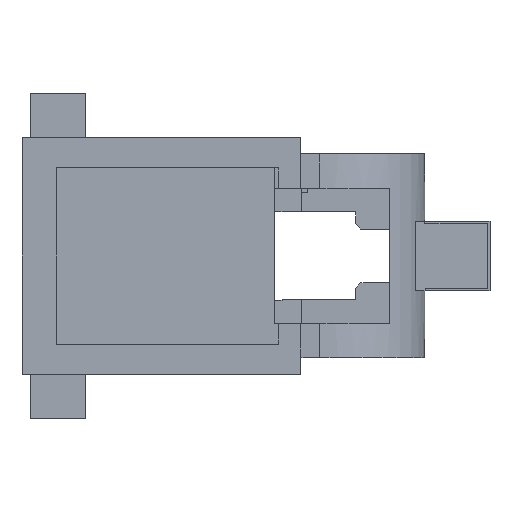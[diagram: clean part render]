
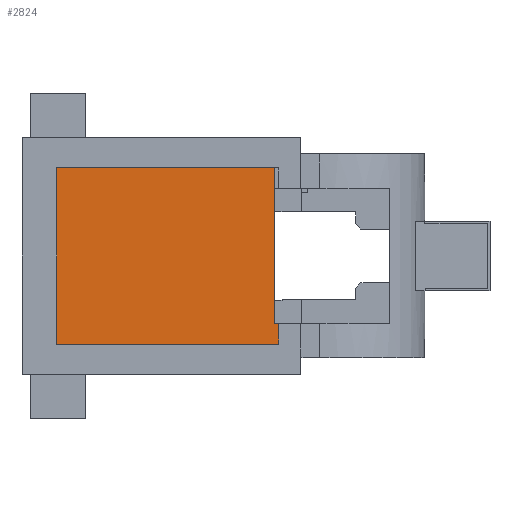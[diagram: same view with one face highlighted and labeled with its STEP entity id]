
A CAD part, left-side view. The second image highlights one B-rep face of the part: STEP entity #2824.
In plain terms, the highlighted planar face has unit normal (-1, 0, 0).
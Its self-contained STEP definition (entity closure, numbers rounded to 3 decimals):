
#642 = PLANE('',#643);
#643 = AXIS2_PLACEMENT_3D('',#644,#645,#646);
#644 = CARTESIAN_POINT('',(-69.606,33.68,21.5));
#645 = DIRECTION('',(0.,-1.,0.));
#646 = DIRECTION('',(1.,0.,0.));
#782 = PLANE('',#783);
#783 = AXIS2_PLACEMENT_3D('',#784,#785,#786);
#784 = CARTESIAN_POINT('',(-177.8,73.213,16.));
#785 = DIRECTION('',(0.,0.,-1.));
#786 = DIRECTION('',(0.,-1.,0.));
#1226 = VERTEX_POINT('',#1227);
#1227 = CARTESIAN_POINT('',(-25.8,33.68,12.218));
#1240 = PLANE('',#1241);
#1241 = AXIS2_PLACEMENT_3D('',#1242,#1243,#1244);
#1242 = CARTESIAN_POINT('',(-177.8,33.7,12.218));
#1243 = DIRECTION('',(0.,0.,-1.));
#1244 = DIRECTION('',(0.,-1.,0.));
#1303 = VERTEX_POINT('',#1304);
#1304 = CARTESIAN_POINT('',(-25.8,33.68,16.));
#1323 = EDGE_CURVE('',#1226,#1303,#1324,.T.);
#1324 = SURFACE_CURVE('',#1325,(#1329,#1335),.PCURVE_S1.);
#1325 = LINE('',#1326,#1327);
#1326 = CARTESIAN_POINT('',(-25.8,33.68,18.75));
#1327 = VECTOR('',#1328,1.);
#1328 = DIRECTION('',(0.,0.,1.));
#1329 = PCURVE('',#642,#1330);
#1330 = DEFINITIONAL_REPRESENTATION('',(#1331),#1334);
#1331 = B_SPLINE_CURVE_WITH_KNOTS('',1,(#1332,#1333),.UNSPECIFIED.,.F.,
  .F.,(2,2),(-7.25,-2.75),.PIECEWISE_BEZIER_KNOTS.);
#1332 = CARTESIAN_POINT('',(43.806,-10.));
#1333 = CARTESIAN_POINT('',(43.806,-5.5));
#1334 = ( GEOMETRIC_REPRESENTATION_CONTEXT(2) 
PARAMETRIC_REPRESENTATION_CONTEXT() REPRESENTATION_CONTEXT('2D SPACE',''
  ) );
#1335 = PCURVE('',#1336,#1341);
#1336 = PLANE('',#1337);
#1337 = AXIS2_PLACEMENT_3D('',#1338,#1339,#1340);
#1338 = CARTESIAN_POINT('',(-25.8,73.213,16.));
#1339 = DIRECTION('',(-1.,0.,0.));
#1340 = DIRECTION('',(0.,0.,-1.));
#1341 = DEFINITIONAL_REPRESENTATION('',(#1342),#1345);
#1342 = B_SPLINE_CURVE_WITH_KNOTS('',1,(#1343,#1344),.UNSPECIFIED.,.F.,
  .F.,(2,2),(-7.25,-2.75),.PIECEWISE_BEZIER_KNOTS.);
#1343 = CARTESIAN_POINT('',(4.5,39.533));
#1344 = CARTESIAN_POINT('',(0.,39.533));
#1345 = ( GEOMETRIC_REPRESENTATION_CONTEXT(2) 
PARAMETRIC_REPRESENTATION_CONTEXT() REPRESENTATION_CONTEXT('2D SPACE',''
  ) );
#1391 = PLANE('',#1392);
#1392 = AXIS2_PLACEMENT_3D('',#1393,#1394,#1395);
#1393 = CARTESIAN_POINT('',(-177.8,73.213,-16.));
#1394 = DIRECTION('',(0.,-1.,0.));
#1395 = DIRECTION('',(0.,0.,1.));
#1419 = PLANE('',#1420);
#1420 = AXIS2_PLACEMENT_3D('',#1421,#1422,#1423);
#1421 = CARTESIAN_POINT('',(-177.8,32.852,-16.));
#1422 = DIRECTION('',(0.,0.,1.));
#1423 = DIRECTION('',(0.,1.,0.));
#1447 = PLANE('',#1448);
#1448 = AXIS2_PLACEMENT_3D('',#1449,#1450,#1451);
#1449 = CARTESIAN_POINT('',(-177.8,32.852,16.));
#1450 = DIRECTION('',(0.,1.,0.));
#1451 = DIRECTION('',(0.,0.,-1.));
#1475 = PLANE('',#1476);
#1476 = AXIS2_PLACEMENT_3D('',#1477,#1478,#1479);
#1477 = CARTESIAN_POINT('',(-177.8,28.825,-12.276));
#1478 = DIRECTION('',(0.,0.,1.));
#1479 = DIRECTION('',(0.,1.,0.));
#1936 = EDGE_CURVE('',#1937,#1303,#1939,.T.);
#1937 = VERTEX_POINT('',#1938);
#1938 = CARTESIAN_POINT('',(-25.8,73.213,16.));
#1939 = SURFACE_CURVE('',#1940,(#1944,#1951),.PCURVE_S1.);
#1940 = LINE('',#1941,#1942);
#1941 = CARTESIAN_POINT('',(-25.8,73.213,16.));
#1942 = VECTOR('',#1943,1.);
#1943 = DIRECTION('',(0.,-1.,0.));
#1944 = PCURVE('',#782,#1945);
#1945 = DEFINITIONAL_REPRESENTATION('',(#1946),#1950);
#1946 = LINE('',#1947,#1948);
#1947 = CARTESIAN_POINT('',(0.,-152.));
#1948 = VECTOR('',#1949,1.);
#1949 = DIRECTION('',(1.,0.));
#1950 = ( GEOMETRIC_REPRESENTATION_CONTEXT(2) 
PARAMETRIC_REPRESENTATION_CONTEXT() REPRESENTATION_CONTEXT('2D SPACE',''
  ) );
#1951 = PCURVE('',#1336,#1952);
#1952 = DEFINITIONAL_REPRESENTATION('',(#1953),#1957);
#1953 = LINE('',#1954,#1955);
#1954 = CARTESIAN_POINT('',(0.,0.));
#1955 = VECTOR('',#1956,1.);
#1956 = DIRECTION('',(0.,1.));
#1957 = ( GEOMETRIC_REPRESENTATION_CONTEXT(2) 
PARAMETRIC_REPRESENTATION_CONTEXT() REPRESENTATION_CONTEXT('2D SPACE',''
  ) );
#2701 = EDGE_CURVE('',#2702,#1226,#2704,.T.);
#2702 = VERTEX_POINT('',#2703);
#2703 = CARTESIAN_POINT('',(-25.8,33.7,12.218));
#2704 = SURFACE_CURVE('',#2705,(#2709,#2715),.PCURVE_S1.);
#2705 = LINE('',#2706,#2707);
#2706 = CARTESIAN_POINT('',(-25.8,53.456,12.218));
#2707 = VECTOR('',#2708,1.);
#2708 = DIRECTION('',(0.,-1.,0.));
#2709 = PCURVE('',#1240,#2710);
#2710 = DEFINITIONAL_REPRESENTATION('',(#2711),#2714);
#2711 = B_SPLINE_CURVE_WITH_KNOTS('',1,(#2712,#2713),.UNSPECIFIED.,.F.,
  .F.,(2,2),(19.756,20.604),.PIECEWISE_BEZIER_KNOTS.);
#2712 = CARTESIAN_POINT('',(0.,-152.));
#2713 = CARTESIAN_POINT('',(0.848,-152.));
#2714 = ( GEOMETRIC_REPRESENTATION_CONTEXT(2) 
PARAMETRIC_REPRESENTATION_CONTEXT() REPRESENTATION_CONTEXT('2D SPACE',''
  ) );
#2715 = PCURVE('',#1336,#2716);
#2716 = DEFINITIONAL_REPRESENTATION('',(#2717),#2720);
#2717 = B_SPLINE_CURVE_WITH_KNOTS('',1,(#2718,#2719),.UNSPECIFIED.,.F.,
  .F.,(2,2),(19.756,20.604),.PIECEWISE_BEZIER_KNOTS.);
#2718 = CARTESIAN_POINT('',(3.782,39.513));
#2719 = CARTESIAN_POINT('',(3.782,40.361));
#2720 = ( GEOMETRIC_REPRESENTATION_CONTEXT(2) 
PARAMETRIC_REPRESENTATION_CONTEXT() REPRESENTATION_CONTEXT('2D SPACE',''
  ) );
#2738 = PLANE('',#2739);
#2739 = AXIS2_PLACEMENT_3D('',#2740,#2741,#2742);
#2740 = CARTESIAN_POINT('',(-177.8,33.7,-12.276));
#2741 = DIRECTION('',(0.,-1.,0.));
#2742 = DIRECTION('',(0.,0.,1.));
#2824 = ADVANCED_FACE('',(#2825),#1336,.T.);
#2825 = FACE_BOUND('',#2826,.T.);
#2826 = EDGE_LOOP('',(#2827,#2828,#2829,#2830,#2853,#2876,#2899,#2920));
#2827 = ORIENTED_EDGE('',*,*,#2701,.T.);
#2828 = ORIENTED_EDGE('',*,*,#1323,.T.);
#2829 = ORIENTED_EDGE('',*,*,#1936,.F.);
#2830 = ORIENTED_EDGE('',*,*,#2831,.F.);
#2831 = EDGE_CURVE('',#2832,#1937,#2834,.T.);
#2832 = VERTEX_POINT('',#2833);
#2833 = CARTESIAN_POINT('',(-25.8,73.213,-16.));
#2834 = SURFACE_CURVE('',#2835,(#2839,#2846),.PCURVE_S1.);
#2835 = LINE('',#2836,#2837);
#2836 = CARTESIAN_POINT('',(-25.8,73.213,-16.));
#2837 = VECTOR('',#2838,1.);
#2838 = DIRECTION('',(0.,0.,1.));
#2839 = PCURVE('',#1336,#2840);
#2840 = DEFINITIONAL_REPRESENTATION('',(#2841),#2845);
#2841 = LINE('',#2842,#2843);
#2842 = CARTESIAN_POINT('',(32.,0.));
#2843 = VECTOR('',#2844,1.);
#2844 = DIRECTION('',(-1.,0.));
#2845 = ( GEOMETRIC_REPRESENTATION_CONTEXT(2) 
PARAMETRIC_REPRESENTATION_CONTEXT() REPRESENTATION_CONTEXT('2D SPACE',''
  ) );
#2846 = PCURVE('',#1391,#2847);
#2847 = DEFINITIONAL_REPRESENTATION('',(#2848),#2852);
#2848 = LINE('',#2849,#2850);
#2849 = CARTESIAN_POINT('',(0.,-152.));
#2850 = VECTOR('',#2851,1.);
#2851 = DIRECTION('',(1.,0.));
#2852 = ( GEOMETRIC_REPRESENTATION_CONTEXT(2) 
PARAMETRIC_REPRESENTATION_CONTEXT() REPRESENTATION_CONTEXT('2D SPACE',''
  ) );
#2853 = ORIENTED_EDGE('',*,*,#2854,.F.);
#2854 = EDGE_CURVE('',#2855,#2832,#2857,.T.);
#2855 = VERTEX_POINT('',#2856);
#2856 = CARTESIAN_POINT('',(-25.8,32.852,-16.));
#2857 = SURFACE_CURVE('',#2858,(#2862,#2869),.PCURVE_S1.);
#2858 = LINE('',#2859,#2860);
#2859 = CARTESIAN_POINT('',(-25.8,32.852,-16.));
#2860 = VECTOR('',#2861,1.);
#2861 = DIRECTION('',(0.,1.,0.));
#2862 = PCURVE('',#1336,#2863);
#2863 = DEFINITIONAL_REPRESENTATION('',(#2864),#2868);
#2864 = LINE('',#2865,#2866);
#2865 = CARTESIAN_POINT('',(32.,40.361));
#2866 = VECTOR('',#2867,1.);
#2867 = DIRECTION('',(0.,-1.));
#2868 = ( GEOMETRIC_REPRESENTATION_CONTEXT(2) 
PARAMETRIC_REPRESENTATION_CONTEXT() REPRESENTATION_CONTEXT('2D SPACE',''
  ) );
#2869 = PCURVE('',#1419,#2870);
#2870 = DEFINITIONAL_REPRESENTATION('',(#2871),#2875);
#2871 = LINE('',#2872,#2873);
#2872 = CARTESIAN_POINT('',(0.,-152.));
#2873 = VECTOR('',#2874,1.);
#2874 = DIRECTION('',(1.,0.));
#2875 = ( GEOMETRIC_REPRESENTATION_CONTEXT(2) 
PARAMETRIC_REPRESENTATION_CONTEXT() REPRESENTATION_CONTEXT('2D SPACE',''
  ) );
#2876 = ORIENTED_EDGE('',*,*,#2877,.F.);
#2877 = EDGE_CURVE('',#2878,#2855,#2880,.T.);
#2878 = VERTEX_POINT('',#2879);
#2879 = CARTESIAN_POINT('',(-25.8,32.852,-12.276));
#2880 = SURFACE_CURVE('',#2881,(#2885,#2892),.PCURVE_S1.);
#2881 = LINE('',#2882,#2883);
#2882 = CARTESIAN_POINT('',(-25.8,32.852,16.));
#2883 = VECTOR('',#2884,1.);
#2884 = DIRECTION('',(0.,0.,-1.));
#2885 = PCURVE('',#1336,#2886);
#2886 = DEFINITIONAL_REPRESENTATION('',(#2887),#2891);
#2887 = LINE('',#2888,#2889);
#2888 = CARTESIAN_POINT('',(0.,40.361));
#2889 = VECTOR('',#2890,1.);
#2890 = DIRECTION('',(1.,0.));
#2891 = ( GEOMETRIC_REPRESENTATION_CONTEXT(2) 
PARAMETRIC_REPRESENTATION_CONTEXT() REPRESENTATION_CONTEXT('2D SPACE',''
  ) );
#2892 = PCURVE('',#1447,#2893);
#2893 = DEFINITIONAL_REPRESENTATION('',(#2894),#2898);
#2894 = LINE('',#2895,#2896);
#2895 = CARTESIAN_POINT('',(0.,-152.));
#2896 = VECTOR('',#2897,1.);
#2897 = DIRECTION('',(1.,0.));
#2898 = ( GEOMETRIC_REPRESENTATION_CONTEXT(2) 
PARAMETRIC_REPRESENTATION_CONTEXT() REPRESENTATION_CONTEXT('2D SPACE',''
  ) );
#2899 = ORIENTED_EDGE('',*,*,#2900,.T.);
#2900 = EDGE_CURVE('',#2878,#2901,#2903,.T.);
#2901 = VERTEX_POINT('',#2902);
#2902 = CARTESIAN_POINT('',(-25.8,33.7,-12.276));
#2903 = SURFACE_CURVE('',#2904,(#2908,#2914),.PCURVE_S1.);
#2904 = LINE('',#2905,#2906);
#2905 = CARTESIAN_POINT('',(-25.8,51.019,-12.276));
#2906 = VECTOR('',#2907,1.);
#2907 = DIRECTION('',(0.,1.,0.));
#2908 = PCURVE('',#1336,#2909);
#2909 = DEFINITIONAL_REPRESENTATION('',(#2910),#2913);
#2910 = B_SPLINE_CURVE_WITH_KNOTS('',1,(#2911,#2912),.UNSPECIFIED.,.F.,
  .F.,(2,2),(-18.167,-17.319),.PIECEWISE_BEZIER_KNOTS.);
#2911 = CARTESIAN_POINT('',(28.276,40.361));
#2912 = CARTESIAN_POINT('',(28.276,39.513));
#2913 = ( GEOMETRIC_REPRESENTATION_CONTEXT(2) 
PARAMETRIC_REPRESENTATION_CONTEXT() REPRESENTATION_CONTEXT('2D SPACE',''
  ) );
#2914 = PCURVE('',#1475,#2915);
#2915 = DEFINITIONAL_REPRESENTATION('',(#2916),#2919);
#2916 = B_SPLINE_CURVE_WITH_KNOTS('',1,(#2917,#2918),.UNSPECIFIED.,.F.,
  .F.,(2,2),(-18.167,-17.319),.PIECEWISE_BEZIER_KNOTS.);
#2917 = CARTESIAN_POINT('',(4.027,-152.));
#2918 = CARTESIAN_POINT('',(4.875,-152.));
#2919 = ( GEOMETRIC_REPRESENTATION_CONTEXT(2) 
PARAMETRIC_REPRESENTATION_CONTEXT() REPRESENTATION_CONTEXT('2D SPACE',''
  ) );
#2920 = ORIENTED_EDGE('',*,*,#2921,.T.);
#2921 = EDGE_CURVE('',#2901,#2702,#2922,.T.);
#2922 = SURFACE_CURVE('',#2923,(#2927,#2933),.PCURVE_S1.);
#2923 = LINE('',#2924,#2925);
#2924 = CARTESIAN_POINT('',(-25.8,33.7,1.862));
#2925 = VECTOR('',#2926,1.);
#2926 = DIRECTION('',(0.,0.,1.));
#2927 = PCURVE('',#1336,#2928);
#2928 = DEFINITIONAL_REPRESENTATION('',(#2929),#2932);
#2929 = B_SPLINE_CURVE_WITH_KNOTS('',1,(#2930,#2931),.UNSPECIFIED.,.F.,
  .F.,(2,2),(-14.138,10.356),.PIECEWISE_BEZIER_KNOTS.);
#2930 = CARTESIAN_POINT('',(28.276,39.513));
#2931 = CARTESIAN_POINT('',(3.782,39.513));
#2932 = ( GEOMETRIC_REPRESENTATION_CONTEXT(2) 
PARAMETRIC_REPRESENTATION_CONTEXT() REPRESENTATION_CONTEXT('2D SPACE',''
  ) );
#2933 = PCURVE('',#2738,#2934);
#2934 = DEFINITIONAL_REPRESENTATION('',(#2935),#2938);
#2935 = B_SPLINE_CURVE_WITH_KNOTS('',1,(#2936,#2937),.UNSPECIFIED.,.F.,
  .F.,(2,2),(-14.138,10.356),.PIECEWISE_BEZIER_KNOTS.);
#2936 = CARTESIAN_POINT('',(0.,-152.));
#2937 = CARTESIAN_POINT('',(24.494,-152.));
#2938 = ( GEOMETRIC_REPRESENTATION_CONTEXT(2) 
PARAMETRIC_REPRESENTATION_CONTEXT() REPRESENTATION_CONTEXT('2D SPACE',''
  ) );
